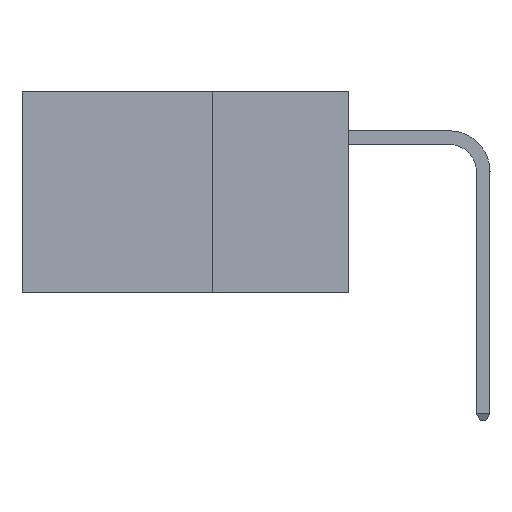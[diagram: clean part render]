
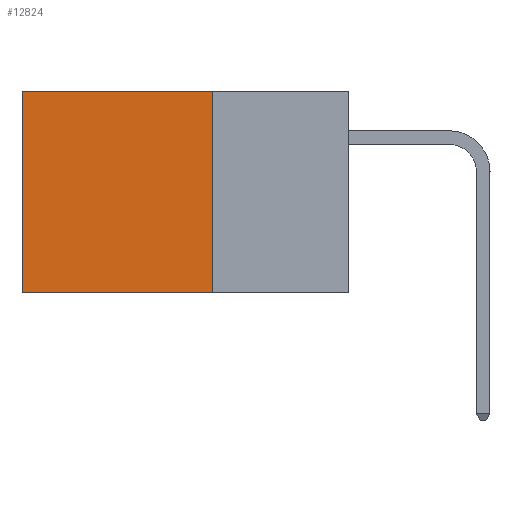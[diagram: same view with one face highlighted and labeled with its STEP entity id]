
A CAD part, left-side view. The second image highlights one B-rep face of the part: STEP entity #12824.
In plain terms, the highlighted planar face has unit normal (-1, 0, 0).
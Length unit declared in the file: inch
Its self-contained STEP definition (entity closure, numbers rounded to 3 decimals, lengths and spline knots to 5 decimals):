
#18 = VERTEX_POINT ( 'NONE', #12216 ) ;
#278 = VECTOR ( 'NONE', #10568, 39.37008 ) ;
#332 = VECTOR ( 'NONE', #9499, 39.37008 ) ;
#502 = LINE ( 'NONE', #13959, #332 ) ;
#506 = LINE ( 'NONE', #5039, #278 ) ;
#575 = CARTESIAN_POINT ( 'NONE',  ( 0.2875, 0.6, -0.37 ) ) ;
#757 = CARTESIAN_POINT ( 'NONE',  ( 0.2875, 0.25, 0. ) ) ;
#1475 = ORIENTED_EDGE ( 'NONE', *, *, #11907, .T. ) ;
#1897 = VERTEX_POINT ( 'NONE', #7597 ) ;
#1966 = AXIS2_PLACEMENT_3D ( 'NONE', #757, #8443, #6059 ) ;
#2275 = EDGE_CURVE ( 'NONE', #3997, #2826, #4065, .T. ) ;
#2309 = CARTESIAN_POINT ( 'NONE',  ( 0.2875, 0.25, -0.37 ) ) ;
#2826 = VERTEX_POINT ( 'NONE', #575 ) ;
#3645 = EDGE_CURVE ( 'NONE', #18, #1897, #12117, .T. ) ;
#3997 = VERTEX_POINT ( 'NONE', #2309 ) ;
#4065 = LINE ( 'NONE', #5624, #8812 ) ;
#5039 = CARTESIAN_POINT ( 'NONE',  ( 0.2875, 0.25, 0. ) ) ;
#5043 = ORIENTED_EDGE ( 'NONE', *, *, #3645, .T. ) ;
#5572 = CARTESIAN_POINT ( 'NONE',  ( 0.2875, 0.25, 0. ) ) ;
#5624 = CARTESIAN_POINT ( 'NONE',  ( 0.2875, 0.25, -0.37 ) ) ;
#5867 = EDGE_LOOP ( 'NONE', ( #1475, #12050, #10010, #5043 ) ) ;
#6059 = DIRECTION ( 'NONE',  ( 0., 0., -1. ) ) ;
#6526 = EDGE_CURVE ( 'NONE', #18, #3997, #506, .T. ) ;
#7207 = PLANE ( 'NONE',  #1966 ) ;
#7597 = CARTESIAN_POINT ( 'NONE',  ( 0.2875, 0.6, 0. ) ) ;
#8443 = DIRECTION ( 'NONE',  ( 1., 0., 0. ) ) ;
#8812 = VECTOR ( 'NONE', #13378, 39.37008 ) ;
#8873 = DIRECTION ( 'NONE',  ( 0., 1., 0. ) ) ;
#8900 = VECTOR ( 'NONE', #8873, 39.37008 ) ;
#9442 = FACE_OUTER_BOUND ( 'NONE', #5867, .T. ) ;
#9499 = DIRECTION ( 'NONE',  ( 0., 0., -1. ) ) ;
#10010 = ORIENTED_EDGE ( 'NONE', *, *, #6526, .F. ) ;
#10568 = DIRECTION ( 'NONE',  ( 0., 0., -1. ) ) ;
#11907 = EDGE_CURVE ( 'NONE', #1897, #2826, #502, .T. ) ;
#12050 = ORIENTED_EDGE ( 'NONE', *, *, #2275, .F. ) ;
#12117 = LINE ( 'NONE', #5572, #8900 ) ;
#12216 = CARTESIAN_POINT ( 'NONE',  ( 0.2875, 0.25, 0. ) ) ;
#12824 = ADVANCED_FACE ( 'NONE', ( #9442 ), #7207, .F. ) ;
#13378 = DIRECTION ( 'NONE',  ( 0., 1., 0. ) ) ;
#13959 = CARTESIAN_POINT ( 'NONE',  ( 0.2875, 0.6, 0. ) ) ;
